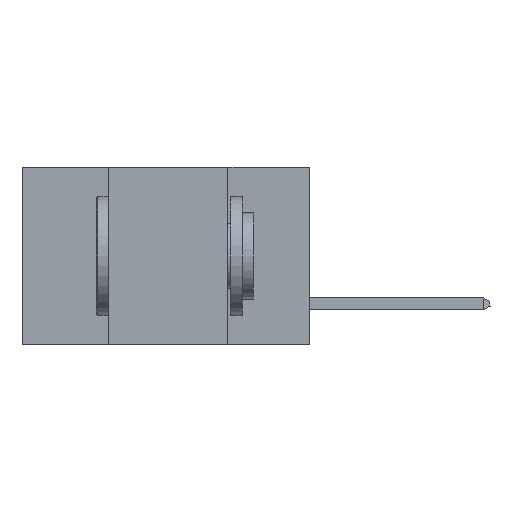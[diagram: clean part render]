
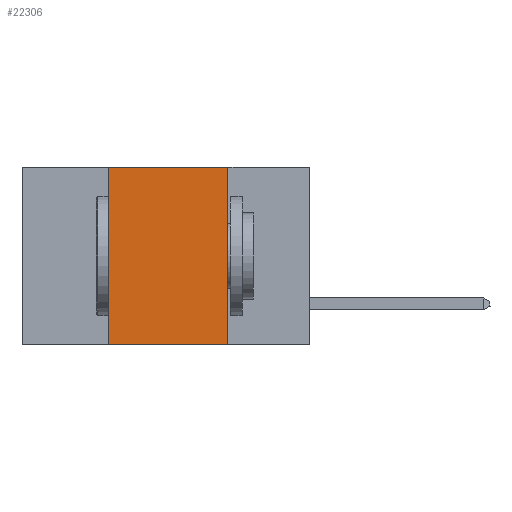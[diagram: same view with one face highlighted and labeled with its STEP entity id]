
A CAD part, left-side view. The second image highlights one B-rep face of the part: STEP entity #22306.
In plain terms, the highlighted planar face has unit normal (-1, 0, 0).
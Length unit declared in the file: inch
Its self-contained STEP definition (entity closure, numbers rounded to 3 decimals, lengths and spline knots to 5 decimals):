
#1650 = VERTEX_POINT ( 'NONE', #28345 ) ;
#3673 = ORIENTED_EDGE ( 'NONE', *, *, #9617, .T. ) ;
#8004 = CARTESIAN_POINT ( 'NONE',  ( 0., 0.17, 0. ) ) ;
#8755 = VERTEX_POINT ( 'NONE', #44941 ) ;
#9617 = EDGE_CURVE ( 'NONE', #37204, #1650, #28960, .T. ) ;
#10167 = DIRECTION ( 'NONE',  ( 0., -1., 0. ) ) ;
#11932 = VECTOR ( 'NONE', #16322, 39.37008 ) ;
#14879 = DIRECTION ( 'NONE',  ( 0., 0., -1. ) ) ;
#16000 = ORIENTED_EDGE ( 'NONE', *, *, #27825, .F. ) ;
#16322 = DIRECTION ( 'NONE',  ( 0., -1., 0. ) ) ;
#16450 = EDGE_CURVE ( 'NONE', #8755, #33075, #25784, .T. ) ;
#16826 = EDGE_CURVE ( 'NONE', #33075, #1650, #25741, .T. ) ;
#17529 = AXIS2_PLACEMENT_3D ( 'NONE', #39072, #18164, #42957 ) ;
#18164 = DIRECTION ( 'NONE',  ( 1., 0., 0. ) ) ;
#19143 = CARTESIAN_POINT ( 'NONE',  ( 0., 0.17, 0. ) ) ;
#22306 = ADVANCED_FACE ( 'NONE', ( #45826 ), #25106, .F. ) ;
#23315 = DIRECTION ( 'NONE',  ( 0., 0., 1. ) ) ;
#25106 = PLANE ( 'NONE',  #17529 ) ;
#25543 = VECTOR ( 'NONE', #23315, 39.37008 ) ;
#25741 = LINE ( 'NONE', #8004, #27956 ) ;
#25784 = LINE ( 'NONE', #30528, #11932 ) ;
#27825 = EDGE_CURVE ( 'NONE', #37204, #8755, #38308, .T. ) ;
#27956 = VECTOR ( 'NONE', #14879, 39.37008 ) ;
#28345 = CARTESIAN_POINT ( 'NONE',  ( 0., 0.17, -0.37 ) ) ;
#28960 = LINE ( 'NONE', #42275, #41744 ) ;
#30528 = CARTESIAN_POINT ( 'NONE',  ( 0., 0.6, 0. ) ) ;
#33075 = VERTEX_POINT ( 'NONE', #19143 ) ;
#33855 = CARTESIAN_POINT ( 'NONE',  ( 0., 0.42, 0. ) ) ;
#35099 = ORIENTED_EDGE ( 'NONE', *, *, #16826, .F. ) ;
#35232 = CARTESIAN_POINT ( 'NONE',  ( 0., 0.42, -0.37 ) ) ;
#37204 = VERTEX_POINT ( 'NONE', #35232 ) ;
#38308 = LINE ( 'NONE', #33855, #25543 ) ;
#39072 = CARTESIAN_POINT ( 'NONE',  ( 0., 0.6, 0. ) ) ;
#39714 = ORIENTED_EDGE ( 'NONE', *, *, #16450, .F. ) ;
#41030 = EDGE_LOOP ( 'NONE', ( #35099, #39714, #16000, #3673 ) ) ;
#41744 = VECTOR ( 'NONE', #10167, 39.37008 ) ;
#42275 = CARTESIAN_POINT ( 'NONE',  ( 0., 0.6, -0.37 ) ) ;
#42957 = DIRECTION ( 'NONE',  ( 0., 0., -1. ) ) ;
#44941 = CARTESIAN_POINT ( 'NONE',  ( 0., 0.42, 0. ) ) ;
#45826 = FACE_OUTER_BOUND ( 'NONE', #41030, .T. ) ;
